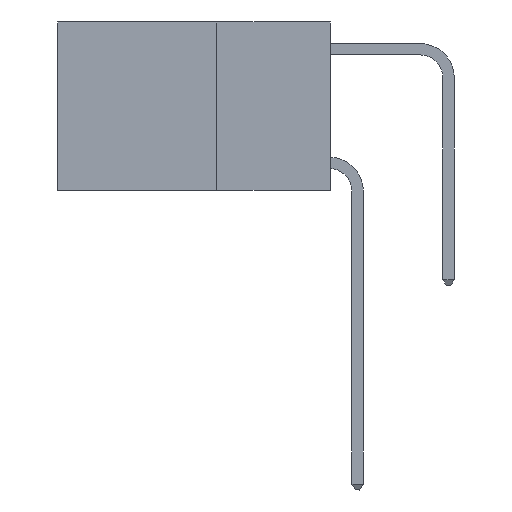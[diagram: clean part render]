
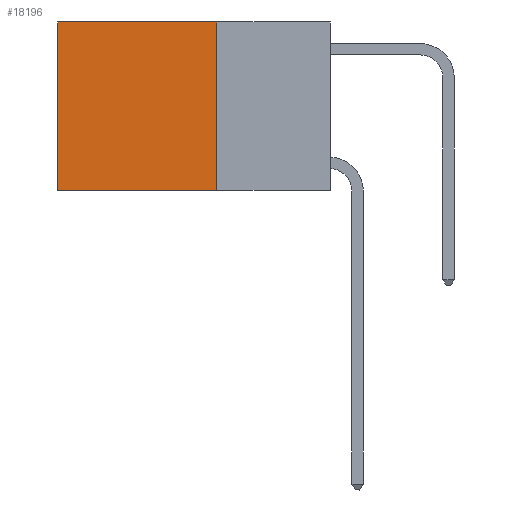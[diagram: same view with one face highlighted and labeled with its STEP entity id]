
A CAD part, left-side view. The second image highlights one B-rep face of the part: STEP entity #18196.
In plain terms, the highlighted planar face has unit normal (-1, 0, 0).
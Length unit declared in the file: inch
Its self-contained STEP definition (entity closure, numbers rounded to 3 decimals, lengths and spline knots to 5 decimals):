
#1515 = EDGE_CURVE ( 'NONE', #16174, #14565, #3724, .T. ) ;
#2592 = DIRECTION ( 'NONE',  ( 0., 0., -1. ) ) ;
#2716 = DIRECTION ( 'NONE',  ( 0., 0., -1. ) ) ;
#3502 = ORIENTED_EDGE ( 'NONE', *, *, #1515, .T. ) ;
#3724 = LINE ( 'NONE', #23280, #21349 ) ;
#4333 = EDGE_CURVE ( 'NONE', #27081, #6775, #23700, .T. ) ;
#4836 = PLANE ( 'NONE',  #15536 ) ;
#4948 = CARTESIAN_POINT ( 'NONE',  ( 0.2625, 0.6, 0. ) ) ;
#5754 = DIRECTION ( 'NONE',  ( 0., 1., 0. ) ) ;
#6273 = ORIENTED_EDGE ( 'NONE', *, *, #16520, .T. ) ;
#6775 = VERTEX_POINT ( 'NONE', #15069 ) ;
#9501 = CARTESIAN_POINT ( 'NONE',  ( 0.2625, 0.25, 0. ) ) ;
#9883 = CARTESIAN_POINT ( 'NONE',  ( 0.2625, 0.25, 0. ) ) ;
#10845 = CARTESIAN_POINT ( 'NONE',  ( 0.2625, 0.25, 0. ) ) ;
#12663 = ORIENTED_EDGE ( 'NONE', *, *, #4333, .F. ) ;
#14488 = DIRECTION ( 'NONE',  ( 0., 0., -1. ) ) ;
#14565 = VERTEX_POINT ( 'NONE', #16394 ) ;
#15069 = CARTESIAN_POINT ( 'NONE',  ( 0.2625, 0.6, -0.37 ) ) ;
#15536 = AXIS2_PLACEMENT_3D ( 'NONE', #9501, #16383, #2592 ) ;
#16174 = VERTEX_POINT ( 'NONE', #10845 ) ;
#16383 = DIRECTION ( 'NONE',  ( 1., 0., 0. ) ) ;
#16394 = CARTESIAN_POINT ( 'NONE',  ( 0.2625, 0.6, 0. ) ) ;
#16520 = EDGE_CURVE ( 'NONE', #14565, #6775, #25300, .T. ) ;
#17498 = EDGE_LOOP ( 'NONE', ( #6273, #12663, #25049, #3502 ) ) ;
#17552 = VECTOR ( 'NONE', #5754, 39.37008 ) ;
#17662 = VECTOR ( 'NONE', #14488, 39.37008 ) ;
#18196 = ADVANCED_FACE ( 'NONE', ( #29491 ), #4836, .F. ) ;
#18692 = DIRECTION ( 'NONE',  ( 0., 1., 0. ) ) ;
#19176 = VECTOR ( 'NONE', #2716, 39.37008 ) ;
#21349 = VECTOR ( 'NONE', #18692, 39.37008 ) ;
#21835 = CARTESIAN_POINT ( 'NONE',  ( 0.2625, 0.25, -0.37 ) ) ;
#22843 = EDGE_CURVE ( 'NONE', #16174, #27081, #23813, .T. ) ;
#23280 = CARTESIAN_POINT ( 'NONE',  ( 0.2625, 0.25, 0. ) ) ;
#23700 = LINE ( 'NONE', #21835, #17552 ) ;
#23813 = LINE ( 'NONE', #9883, #17662 ) ;
#25049 = ORIENTED_EDGE ( 'NONE', *, *, #22843, .F. ) ;
#25300 = LINE ( 'NONE', #4948, #19176 ) ;
#27081 = VERTEX_POINT ( 'NONE', #29013 ) ;
#29013 = CARTESIAN_POINT ( 'NONE',  ( 0.2625, 0.25, -0.37 ) ) ;
#29491 = FACE_OUTER_BOUND ( 'NONE', #17498, .T. ) ;
